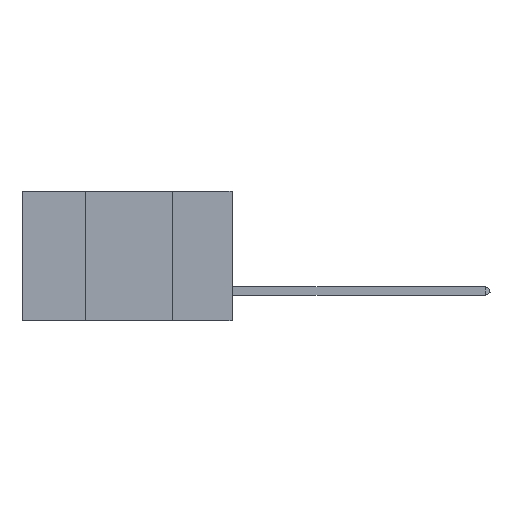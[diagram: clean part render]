
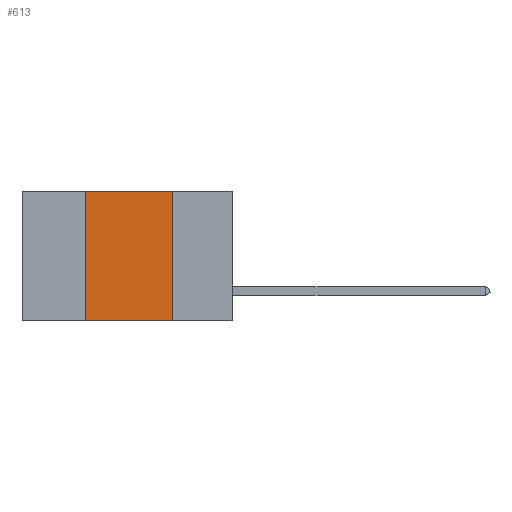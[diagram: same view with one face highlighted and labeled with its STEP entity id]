
A CAD part, left-side view. The second image highlights one B-rep face of the part: STEP entity #613.
In plain terms, the highlighted planar face has unit normal (-1, 0, 0).
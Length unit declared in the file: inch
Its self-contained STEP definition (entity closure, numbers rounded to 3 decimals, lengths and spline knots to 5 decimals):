
#444 = VECTOR ( 'NONE', #20048, 39.37008 ) ;
#613 = ADVANCED_FACE ( 'NONE', ( #2657 ), #8726, .F. ) ;
#1692 = EDGE_LOOP ( 'NONE', ( #18387, #18358, #18480, #25317 ) ) ;
#2657 = FACE_OUTER_BOUND ( 'NONE', #1692, .T. ) ;
#2842 = LINE ( 'NONE', #9175, #19779 ) ;
#4520 = EDGE_CURVE ( 'NONE', #10754, #9616, #18051, .T. ) ;
#4760 = DIRECTION ( 'NONE',  ( 0., -1., 0. ) ) ;
#5197 = CARTESIAN_POINT ( 'NONE',  ( 0., 0.42, -0.37 ) ) ;
#7356 = CARTESIAN_POINT ( 'NONE',  ( 0., 0.6, -0.37 ) ) ;
#8039 = VERTEX_POINT ( 'NONE', #5197 ) ;
#8726 = PLANE ( 'NONE',  #16337 ) ;
#9175 = CARTESIAN_POINT ( 'NONE',  ( 0., 0.6, 0. ) ) ;
#9616 = VERTEX_POINT ( 'NONE', #18408 ) ;
#9674 = LINE ( 'NONE', #26088, #24689 ) ;
#10754 = VERTEX_POINT ( 'NONE', #20490 ) ;
#10935 = CARTESIAN_POINT ( 'NONE',  ( 0., 0.6, 0. ) ) ;
#11664 = LINE ( 'NONE', #7356, #444 ) ;
#12341 = VECTOR ( 'NONE', #19991, 39.37008 ) ;
#13526 = CARTESIAN_POINT ( 'NONE',  ( 0., 0.17, 0. ) ) ;
#15296 = VERTEX_POINT ( 'NONE', #24905 ) ;
#16337 = AXIS2_PLACEMENT_3D ( 'NONE', #10935, #21419, #25956 ) ;
#18051 = LINE ( 'NONE', #13526, #12341 ) ;
#18077 = DIRECTION ( 'NONE',  ( 0., 0., 1. ) ) ;
#18358 = ORIENTED_EDGE ( 'NONE', *, *, #23765, .F. ) ;
#18387 = ORIENTED_EDGE ( 'NONE', *, *, #4520, .F. ) ;
#18408 = CARTESIAN_POINT ( 'NONE',  ( 0., 0.17, -0.37 ) ) ;
#18480 = ORIENTED_EDGE ( 'NONE', *, *, #26682, .F. ) ;
#19779 = VECTOR ( 'NONE', #4760, 39.37008 ) ;
#19991 = DIRECTION ( 'NONE',  ( 0., 0., -1. ) ) ;
#20048 = DIRECTION ( 'NONE',  ( 0., -1., 0. ) ) ;
#20490 = CARTESIAN_POINT ( 'NONE',  ( 0., 0.17, 0. ) ) ;
#21419 = DIRECTION ( 'NONE',  ( 1., 0., 0. ) ) ;
#23765 = EDGE_CURVE ( 'NONE', #15296, #10754, #2842, .T. ) ;
#24689 = VECTOR ( 'NONE', #18077, 39.37008 ) ;
#24905 = CARTESIAN_POINT ( 'NONE',  ( 0., 0.42, 0. ) ) ;
#25317 = ORIENTED_EDGE ( 'NONE', *, *, #26308, .T. ) ;
#25956 = DIRECTION ( 'NONE',  ( 0., 0., -1. ) ) ;
#26088 = CARTESIAN_POINT ( 'NONE',  ( 0., 0.42, 0. ) ) ;
#26308 = EDGE_CURVE ( 'NONE', #8039, #9616, #11664, .T. ) ;
#26682 = EDGE_CURVE ( 'NONE', #8039, #15296, #9674, .T. ) ;
